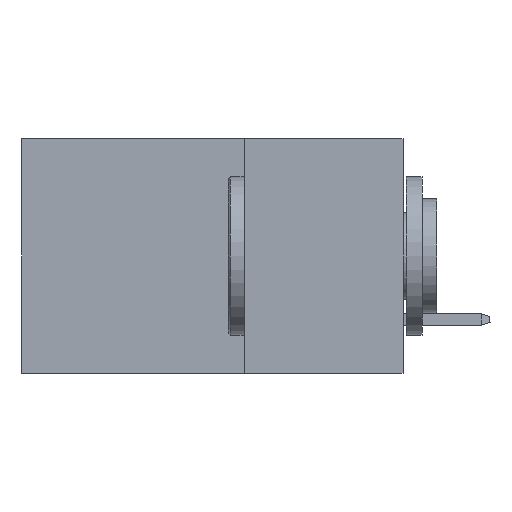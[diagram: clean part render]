
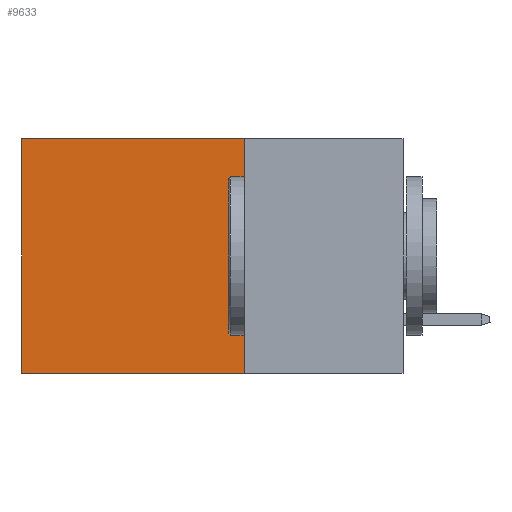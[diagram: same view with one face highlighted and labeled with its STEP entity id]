
A CAD part, left-side view. The second image highlights one B-rep face of the part: STEP entity #9633.
In plain terms, the highlighted planar face has unit normal (-1, 0, 0).
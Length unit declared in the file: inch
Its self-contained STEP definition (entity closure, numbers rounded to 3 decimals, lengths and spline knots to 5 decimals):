
#751 = CARTESIAN_POINT ( 'NONE',  ( 0.2875, 0.6, 0. ) ) ;
#969 = DIRECTION ( 'NONE',  ( 0., 1., 0. ) ) ;
#1953 = VECTOR ( 'NONE', #12828, 39.37008 ) ;
#3184 = VERTEX_POINT ( 'NONE', #751 ) ;
#3717 = EDGE_CURVE ( 'NONE', #16478, #26282, #21608, .T. ) ;
#4306 = CARTESIAN_POINT ( 'NONE',  ( 0.2875, 0.25, 0. ) ) ;
#5575 = LINE ( 'NONE', #15063, #38754 ) ;
#5888 = CARTESIAN_POINT ( 'NONE',  ( 0.2875, 0.25, 0. ) ) ;
#6194 = EDGE_CURVE ( 'NONE', #26282, #24437, #34619, .T. ) ;
#6320 = DIRECTION ( 'NONE',  ( 1., 0., 0. ) ) ;
#9197 = PLANE ( 'NONE',  #12587 ) ;
#9302 = CARTESIAN_POINT ( 'NONE',  ( 0.2875, 0.6, 0. ) ) ;
#9523 = ORIENTED_EDGE ( 'NONE', *, *, #6194, .F. ) ;
#9633 = ADVANCED_FACE ( 'NONE', ( #36452 ), #9197, .F. ) ;
#9960 = LINE ( 'NONE', #9302, #1953 ) ;
#12587 = AXIS2_PLACEMENT_3D ( 'NONE', #5888, #6320, #12723 ) ;
#12633 = DIRECTION ( 'NONE',  ( 0., 1., 0. ) ) ;
#12723 = DIRECTION ( 'NONE',  ( 0., 0., -1. ) ) ;
#12828 = DIRECTION ( 'NONE',  ( 0., 0., -1. ) ) ;
#15063 = CARTESIAN_POINT ( 'NONE',  ( 0.2875, 0.25, 0. ) ) ;
#15501 = VECTOR ( 'NONE', #969, 39.37008 ) ;
#15911 = VECTOR ( 'NONE', #41378, 39.37008 ) ;
#16478 = VERTEX_POINT ( 'NONE', #4306 ) ;
#17256 = EDGE_CURVE ( 'NONE', #3184, #24437, #9960, .T. ) ;
#20422 = CARTESIAN_POINT ( 'NONE',  ( 0.2875, 0.25, -0.37 ) ) ;
#20470 = CARTESIAN_POINT ( 'NONE',  ( 0.2875, 0.6, -0.37 ) ) ;
#21608 = LINE ( 'NONE', #34993, #15911 ) ;
#22943 = EDGE_CURVE ( 'NONE', #16478, #3184, #5575, .T. ) ;
#23718 = ORIENTED_EDGE ( 'NONE', *, *, #3717, .F. ) ;
#24437 = VERTEX_POINT ( 'NONE', #20470 ) ;
#26282 = VERTEX_POINT ( 'NONE', #20422 ) ;
#31758 = EDGE_LOOP ( 'NONE', ( #32738, #9523, #23718, #39003 ) ) ;
#32738 = ORIENTED_EDGE ( 'NONE', *, *, #17256, .T. ) ;
#34619 = LINE ( 'NONE', #41013, #15501 ) ;
#34993 = CARTESIAN_POINT ( 'NONE',  ( 0.2875, 0.25, 0. ) ) ;
#36452 = FACE_OUTER_BOUND ( 'NONE', #31758, .T. ) ;
#38754 = VECTOR ( 'NONE', #12633, 39.37008 ) ;
#39003 = ORIENTED_EDGE ( 'NONE', *, *, #22943, .T. ) ;
#41013 = CARTESIAN_POINT ( 'NONE',  ( 0.2875, 0.25, -0.37 ) ) ;
#41378 = DIRECTION ( 'NONE',  ( 0., 0., -1. ) ) ;
